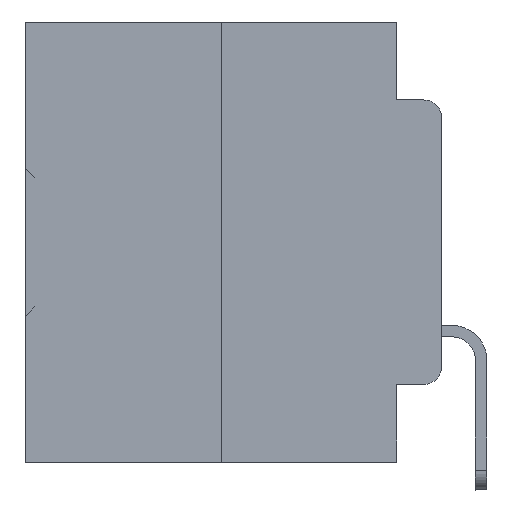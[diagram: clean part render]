
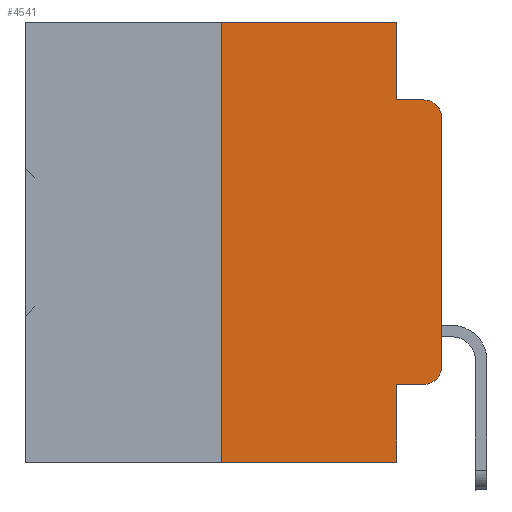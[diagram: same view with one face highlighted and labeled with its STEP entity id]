
A CAD part, left-side view. The second image highlights one B-rep face of the part: STEP entity #4541.
In plain terms, the highlighted planar face has unit normal (-1, 0, 0).
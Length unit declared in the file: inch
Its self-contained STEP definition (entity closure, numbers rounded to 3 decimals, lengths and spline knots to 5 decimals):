
#409 = VERTEX_POINT ( 'NONE', #11731 ) ;
#1268 = DIRECTION ( 'NONE',  ( 0., 0., -1. ) ) ;
#1547 = VECTOR ( 'NONE', #6192, 39.37008 ) ;
#2170 = DIRECTION ( 'NONE',  ( 0., 0., -1. ) ) ;
#2417 = ORIENTED_EDGE ( 'NONE', *, *, #31871, .F. ) ;
#2791 = LINE ( 'NONE', #11025, #3908 ) ;
#2993 = CARTESIAN_POINT ( 'NONE',  ( 0., 0.051, -0.4115 ) ) ;
#3908 = VECTOR ( 'NONE', #14761, 39.37008 ) ;
#4541 = ADVANCED_FACE ( 'NONE', ( #34208 ), #19135, .F. ) ;
#5019 = DIRECTION ( 'NONE',  ( 0., -1., 0. ) ) ;
#5499 = DIRECTION ( 'NONE',  ( -1., 0., 0. ) ) ;
#6000 = CARTESIAN_POINT ( 'NONE',  ( 0., 0.25, 0. ) ) ;
#6141 = VECTOR ( 'NONE', #10894, 39.37008 ) ;
#6192 = DIRECTION ( 'NONE',  ( 0., 0., 1. ) ) ;
#6349 = ORIENTED_EDGE ( 'NONE', *, *, #26858, .F. ) ;
#6776 = CARTESIAN_POINT ( 'NONE',  ( 0., 0.051, 0. ) ) ;
#7673 = EDGE_CURVE ( 'NONE', #15545, #14124, #24210, .T. ) ;
#7982 = LINE ( 'NONE', #19923, #12236 ) ;
#7989 = VERTEX_POINT ( 'NONE', #16480 ) ;
#8803 = EDGE_CURVE ( 'NONE', #20177, #34111, #23229, .T. ) ;
#10126 = DIRECTION ( 'NONE',  ( 1., 0., 0. ) ) ;
#10281 = CIRCLE ( 'NONE', #15900, 0.02 ) ;
#10451 = CARTESIAN_POINT ( 'NONE',  ( 0., 0.051, -0.4115 ) ) ;
#10700 = CARTESIAN_POINT ( 'NONE',  ( 0., 0.473, 0. ) ) ;
#10894 = DIRECTION ( 'NONE',  ( 0., -1., 0. ) ) ;
#11025 = CARTESIAN_POINT ( 'NONE',  ( 0., 0.051, -0.0885 ) ) ;
#11731 = CARTESIAN_POINT ( 'NONE',  ( 0., 0.051, -0.0885 ) ) ;
#12144 = CARTESIAN_POINT ( 'NONE',  ( 0., 0.02, -0.0885 ) ) ;
#12236 = VECTOR ( 'NONE', #37741, 39.37008 ) ;
#12453 = CARTESIAN_POINT ( 'NONE',  ( 0., 0.051, 0. ) ) ;
#12734 = ORIENTED_EDGE ( 'NONE', *, *, #16099, .T. ) ;
#13118 = CARTESIAN_POINT ( 'NONE',  ( 0., 0.02, -0.1085 ) ) ;
#13620 = AXIS2_PLACEMENT_3D ( 'NONE', #10700, #10126, #22645 ) ;
#13635 = CARTESIAN_POINT ( 'NONE',  ( 0., 0.25, 0. ) ) ;
#13719 = ORIENTED_EDGE ( 'NONE', *, *, #14712, .T. ) ;
#14124 = VERTEX_POINT ( 'NONE', #13635 ) ;
#14645 = VERTEX_POINT ( 'NONE', #35714 ) ;
#14712 = EDGE_CURVE ( 'NONE', #14645, #37474, #10281, .T. ) ;
#14761 = DIRECTION ( 'NONE',  ( 0., -1., 0. ) ) ;
#15365 = ORIENTED_EDGE ( 'NONE', *, *, #8803, .T. ) ;
#15412 = LINE ( 'NONE', #6776, #28070 ) ;
#15545 = VERTEX_POINT ( 'NONE', #35577 ) ;
#15900 = AXIS2_PLACEMENT_3D ( 'NONE', #13118, #31125, #34063 ) ;
#15969 = VERTEX_POINT ( 'NONE', #2993 ) ;
#16099 = EDGE_CURVE ( 'NONE', #34111, #14645, #7982, .T. ) ;
#16480 = CARTESIAN_POINT ( 'NONE',  ( 0., 0.051, -0.5 ) ) ;
#16962 = VECTOR ( 'NONE', #38035, 39.37008 ) ;
#18529 = ORIENTED_EDGE ( 'NONE', *, *, #22132, .T. ) ;
#19047 = ORIENTED_EDGE ( 'NONE', *, *, #38127, .F. ) ;
#19135 = PLANE ( 'NONE',  #13620 ) ;
#19923 = CARTESIAN_POINT ( 'NONE',  ( 0., 0., 0. ) ) ;
#19941 = ORIENTED_EDGE ( 'NONE', *, *, #31865, .T. ) ;
#20177 = VERTEX_POINT ( 'NONE', #29908 ) ;
#20382 = CARTESIAN_POINT ( 'NONE',  ( 0., 0.051, 0. ) ) ;
#22132 = EDGE_CURVE ( 'NONE', #15969, #20177, #34724, .T. ) ;
#22645 = DIRECTION ( 'NONE',  ( 0., 0., -1. ) ) ;
#22677 = CARTESIAN_POINT ( 'NONE',  ( 0., 0., -0.3915 ) ) ;
#22851 = CARTESIAN_POINT ( 'NONE',  ( 0., 0.473, 0. ) ) ;
#23229 = CIRCLE ( 'NONE', #28886, 0.02 ) ;
#24210 = LINE ( 'NONE', #6000, #1547 ) ;
#25797 = LINE ( 'NONE', #22851, #31771 ) ;
#26675 = CARTESIAN_POINT ( 'NONE',  ( 0., 0.02, -0.3915 ) ) ;
#26858 = EDGE_CURVE ( 'NONE', #15969, #7989, #27537, .T. ) ;
#27537 = LINE ( 'NONE', #12453, #29075 ) ;
#27885 = EDGE_LOOP ( 'NONE', ( #12734, #13719, #19047, #37617, #2417, #32166, #19941, #6349, #18529, #15365 ) ) ;
#28070 = VECTOR ( 'NONE', #1268, 39.37008 ) ;
#28886 = AXIS2_PLACEMENT_3D ( 'NONE', #26675, #5499, #2170 ) ;
#29075 = VECTOR ( 'NONE', #34170, 39.37008 ) ;
#29908 = CARTESIAN_POINT ( 'NONE',  ( 0., 0.02, -0.4115 ) ) ;
#31125 = DIRECTION ( 'NONE',  ( -1., 0., 0. ) ) ;
#31285 = LINE ( 'NONE', #37920, #6141 ) ;
#31771 = VECTOR ( 'NONE', #5019, 39.37008 ) ;
#31865 = EDGE_CURVE ( 'NONE', #15545, #7989, #31285, .T. ) ;
#31871 = EDGE_CURVE ( 'NONE', #14124, #37210, #25797, .T. ) ;
#32166 = ORIENTED_EDGE ( 'NONE', *, *, #7673, .F. ) ;
#32657 = EDGE_CURVE ( 'NONE', #37210, #409, #15412, .T. ) ;
#34063 = DIRECTION ( 'NONE',  ( 0., 0., -1. ) ) ;
#34111 = VERTEX_POINT ( 'NONE', #22677 ) ;
#34170 = DIRECTION ( 'NONE',  ( 0., 0., -1. ) ) ;
#34208 = FACE_OUTER_BOUND ( 'NONE', #27885, .T. ) ;
#34724 = LINE ( 'NONE', #10451, #16962 ) ;
#35577 = CARTESIAN_POINT ( 'NONE',  ( 0., 0.25, -0.5 ) ) ;
#35714 = CARTESIAN_POINT ( 'NONE',  ( 0., 0., -0.1085 ) ) ;
#37210 = VERTEX_POINT ( 'NONE', #20382 ) ;
#37474 = VERTEX_POINT ( 'NONE', #12144 ) ;
#37617 = ORIENTED_EDGE ( 'NONE', *, *, #32657, .F. ) ;
#37741 = DIRECTION ( 'NONE',  ( 0., 0., 1. ) ) ;
#37920 = CARTESIAN_POINT ( 'NONE',  ( 0., 0.473, -0.5 ) ) ;
#38035 = DIRECTION ( 'NONE',  ( 0., -1., 0. ) ) ;
#38127 = EDGE_CURVE ( 'NONE', #409, #37474, #2791, .T. ) ;
